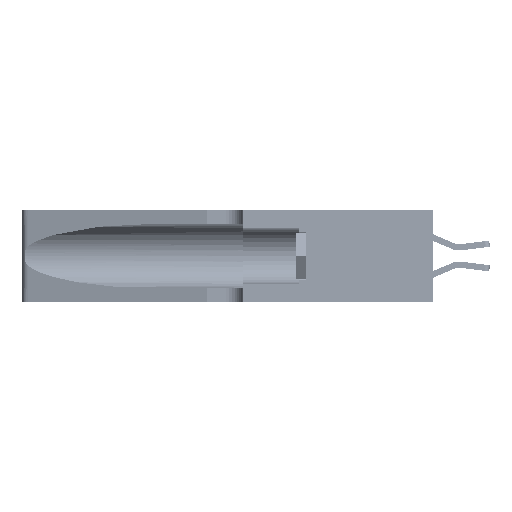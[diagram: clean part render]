
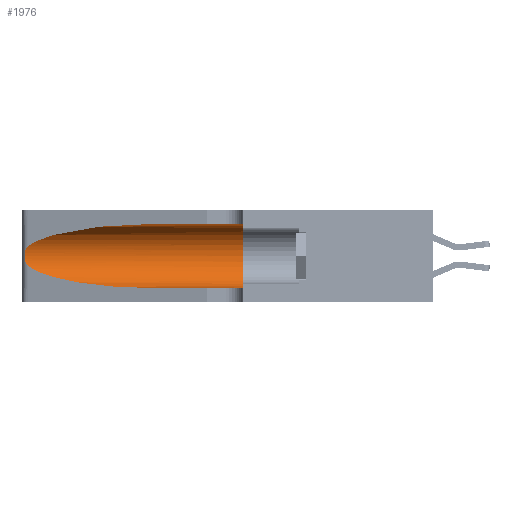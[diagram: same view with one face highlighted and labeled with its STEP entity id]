
A CAD part, left-side view. The second image highlights one B-rep face of the part: STEP entity #1976.
In plain terms, the highlighted cylindrical face has radius 3.308 mm (diameter 6.617 mm), a partial arc.
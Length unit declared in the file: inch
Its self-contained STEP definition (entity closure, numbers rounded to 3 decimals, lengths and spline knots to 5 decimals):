
#940 = VERTEX_POINT ( 'NONE', #50355 ) ;
#1334 = CARTESIAN_POINT ( 'NONE',  ( 0.1305, 1.61858, 0.05475 ) ) ;
#1976 = ADVANCED_FACE ( 'NONE', ( #34396 ), #10896, .F. ) ;
#1998 = EDGE_LOOP ( 'NONE', ( #29993, #45578, #25538, #46905, #43366, #34392 ) ) ;
#2855 = CARTESIAN_POINT ( 'NONE',  ( 0.25639, 1.23186, 0.15144 ) ) ;
#3407 = VERTEX_POINT ( 'NONE', #19071 ) ;
#4101 = CARTESIAN_POINT ( 'NONE',  ( 0.1305, 0.72297, 0.31525 ) ) ;
#4581 = EDGE_CURVE ( 'NONE', #39715, #8170, #14605, .T. ) ;
#4950 = CARTESIAN_POINT ( 'NONE',  ( 0.1305, 0.35, 0.31525 ) ) ;
#5104 = CARTESIAN_POINT ( 'NONE',  ( 0.18966, 0.96281, 0.31525 ) ) ;
#5500 = LINE ( 'NONE', #1334, #37495 ) ;
#5562 = DIRECTION ( 'NONE',  ( 0., -1., 0. ) ) ;
#6789 = CIRCLE ( 'NONE', #49412, 0.13025 ) ;
#7079 = CARTESIAN_POINT ( 'NONE',  ( 0.25487, 1.22718, 0.14631 ) ) ;
#7545 = CARTESIAN_POINT ( 'NONE',  ( 0.1305, 0.72297, 0.05475 ) ) ;
#8170 = VERTEX_POINT ( 'NONE', #4950 ) ;
#9162 = EDGE_CURVE ( 'NONE', #39859, #940, #10877, .T. ) ;
#10358 = VERTEX_POINT ( 'NONE', #20147 ) ;
#10721 = EDGE_CURVE ( 'NONE', #940, #10358, #5500, .T. ) ;
#10877 =( BOUNDED_CURVE ( )  B_SPLINE_CURVE ( 3, ( #53011, #40689, #32602, #7545 ),
 .UNSPECIFIED., .F., .F. ) 
 B_SPLINE_CURVE_WITH_KNOTS ( ( 4, 4 ),
 ( 3.44316, 4.71239 ),
 .UNSPECIFIED. ) 
 CURVE ( )  GEOMETRIC_REPRESENTATION_ITEM ( )  RATIONAL_B_SPLINE_CURVE ( ( 1., 0.87, 0.87, 1. ) ) 
 REPRESENTATION_ITEM ( '' )  );
#10896 = CYLINDRICAL_SURFACE ( 'NONE', #17068, 0.13025 ) ;
#11111 = CARTESIAN_POINT ( 'NONE',  ( 0.25639, 1.23184, 0.21858 ) ) ;
#11930 = CARTESIAN_POINT ( 'NONE',  ( 0.25487, 1.22718, 0.14631 ) ) ;
#12854 = CARTESIAN_POINT ( 'NONE',  ( 0.1305, 0.35, 0.185 ) ) ;
#14605 = LINE ( 'NONE', #22237, #46364 ) ;
#15177 = CARTESIAN_POINT ( 'NONE',  ( 0.25487, 1.22718, 0.22369 ) ) ;
#15366 = CARTESIAN_POINT ( 'NONE',  ( 0.25854, 1.2359, 0.20912 ) ) ;
#17068 = AXIS2_PLACEMENT_3D ( 'NONE', #53098, #49021, #24371 ) ;
#17105 = DIRECTION ( 'NONE',  ( 0., 0., 1. ) ) ;
#17838 = CARTESIAN_POINT ( 'NONE',  ( 0.2373, 1.15595, 0.28018 ) ) ;
#19071 = CARTESIAN_POINT ( 'NONE',  ( 0.25487, 1.22718, 0.22369 ) ) ;
#19614 = CARTESIAN_POINT ( 'NONE',  ( 0.26075, 1.23896, 0.19203 ) ) ;
#19916 = EDGE_CURVE ( 'NONE', #8170, #10358, #6789, .T. ) ;
#20147 = CARTESIAN_POINT ( 'NONE',  ( 0.1305, 0.35, 0.05475 ) ) ;
#22237 = CARTESIAN_POINT ( 'NONE',  ( 0.1305, 1.61858, 0.31525 ) ) ;
#23637 = CARTESIAN_POINT ( 'NONE',  ( 0.25555, 1.22994, 0.2215 ) ) ;
#23812 = CARTESIAN_POINT ( 'NONE',  ( 0.26017, 1.23833, 0.17102 ) ) ;
#24371 = DIRECTION ( 'NONE',  ( 0., 0., -1. ) ) ;
#25538 = ORIENTED_EDGE ( 'NONE', *, *, #9162, .T. ) ;
#26272 = DIRECTION ( 'NONE',  ( 0., -1., 0. ) ) ;
#28011 = CARTESIAN_POINT ( 'NONE',  ( 0.25789, 1.23486, 0.15765 ) ) ;
#28629 = EDGE_CURVE ( 'NONE', #39715, #3407, #48750, .T. ) ;
#28917 = EDGE_CURVE ( 'NONE', #3407, #39859, #41468, .T. ) ;
#29993 = ORIENTED_EDGE ( 'NONE', *, *, #28629, .T. ) ;
#32156 = CARTESIAN_POINT ( 'NONE',  ( 0.25555, 1.22993, 0.14849 ) ) ;
#32602 = CARTESIAN_POINT ( 'NONE',  ( 0.18966, 0.96281, 0.05475 ) ) ;
#34294 = CARTESIAN_POINT ( 'NONE',  ( 0.1305, 0.72297, 0.31525 ) ) ;
#34392 = ORIENTED_EDGE ( 'NONE', *, *, #4581, .F. ) ;
#34396 = FACE_OUTER_BOUND ( 'NONE', #1998, .T. ) ;
#37495 = VECTOR ( 'NONE', #5562, 39.37008 ) ;
#39715 = VERTEX_POINT ( 'NONE', #4101 ) ;
#39859 = VERTEX_POINT ( 'NONE', #11930 ) ;
#40237 = CARTESIAN_POINT ( 'NONE',  ( 0.25787, 1.23484, 0.2124 ) ) ;
#40689 = CARTESIAN_POINT ( 'NONE',  ( 0.2373, 1.15595, 0.08982 ) ) ;
#41468 = B_SPLINE_CURVE_WITH_KNOTS ( 'NONE', 3,
 ( #15177, #23637, #11111, #40237, #15366, #44356, #19614, #48483, #23812, #52568, #28011, #2855, #32156, #7079 ),
 .UNSPECIFIED., .F., .F.,
 ( 4, 2, 2, 2, 2, 2, 4 ),
 ( 0., 0.00027, 0.00053, 0.00107, 0.0016, 0.00187, 0.00214 ),
 .UNSPECIFIED. ) ;
#41912 = DIRECTION ( 'NONE',  ( 0., 1., 0. ) ) ;
#43366 = ORIENTED_EDGE ( 'NONE', *, *, #19916, .F. ) ;
#44356 = CARTESIAN_POINT ( 'NONE',  ( 0.26018, 1.23835, 0.19895 ) ) ;
#45578 = ORIENTED_EDGE ( 'NONE', *, *, #28917, .T. ) ;
#46364 = VECTOR ( 'NONE', #26272, 39.37008 ) ;
#46745 = CARTESIAN_POINT ( 'NONE',  ( 0.25487, 1.22718, 0.22369 ) ) ;
#46905 = ORIENTED_EDGE ( 'NONE', *, *, #10721, .T. ) ;
#48483 = CARTESIAN_POINT ( 'NONE',  ( 0.26075, 1.23896, 0.178 ) ) ;
#48750 =( BOUNDED_CURVE ( )  B_SPLINE_CURVE ( 3, ( #34294, #5104, #17838, #46745 ),
 .UNSPECIFIED., .F., .T. ) 
 B_SPLINE_CURVE_WITH_KNOTS ( ( 4, 4 ),
 ( 1.5708, 2.84003 ),
 .UNSPECIFIED. ) 
 CURVE ( )  GEOMETRIC_REPRESENTATION_ITEM ( )  RATIONAL_B_SPLINE_CURVE ( ( 1., 0.87, 0.87, 1. ) ) 
 REPRESENTATION_ITEM ( '' )  );
#49021 = DIRECTION ( 'NONE',  ( 0., -1., 0. ) ) ;
#49412 = AXIS2_PLACEMENT_3D ( 'NONE', #12854, #41912, #17105 ) ;
#50355 = CARTESIAN_POINT ( 'NONE',  ( 0.1305, 0.72297, 0.05475 ) ) ;
#52568 = CARTESIAN_POINT ( 'NONE',  ( 0.25856, 1.23593, 0.16098 ) ) ;
#53011 = CARTESIAN_POINT ( 'NONE',  ( 0.25487, 1.22718, 0.14631 ) ) ;
#53098 = CARTESIAN_POINT ( 'NONE',  ( 0.1305, 1.61858, 0.185 ) ) ;
